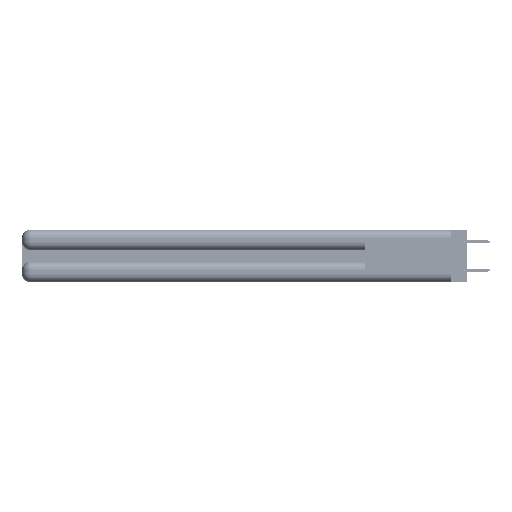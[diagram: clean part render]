
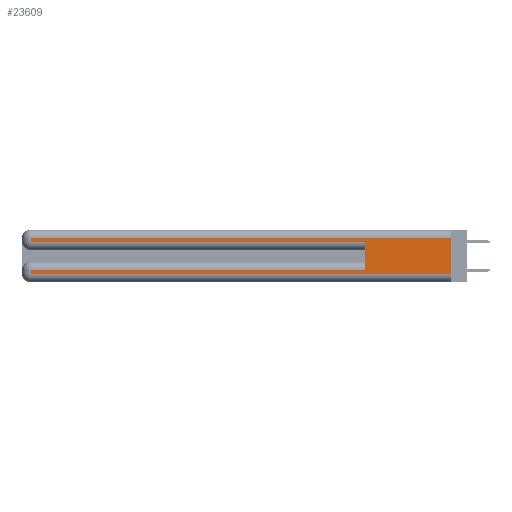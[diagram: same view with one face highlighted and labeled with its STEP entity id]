
A CAD part, left-side view. The second image highlights one B-rep face of the part: STEP entity #23609.
In plain terms, the highlighted planar face has unit normal (-1, 0, 0).
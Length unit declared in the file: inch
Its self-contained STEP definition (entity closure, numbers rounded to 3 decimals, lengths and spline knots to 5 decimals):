
#716 = DIRECTION ( 'NONE',  ( 0., 1., 0. ) ) ;
#971 = VECTOR ( 'NONE', #18711, 39.37008 ) ;
#2252 = LINE ( 'NONE', #43700, #971 ) ;
#2614 = CARTESIAN_POINT ( 'NONE',  ( 0., 0., 0.37 ) ) ;
#4484 = ORIENTED_EDGE ( 'NONE', *, *, #27002, .T. ) ;
#5103 = DIRECTION ( 'NONE',  ( 0., 0., -1. ) ) ;
#5315 = EDGE_CURVE ( 'NONE', #48750, #21793, #53080, .T. ) ;
#6388 = ORIENTED_EDGE ( 'NONE', *, *, #23982, .F. ) ;
#6727 = CARTESIAN_POINT ( 'NONE',  ( 0., 2.94, 0.285 ) ) ;
#11381 = DIRECTION ( 'NONE',  ( 0., 0., 1. ) ) ;
#13896 = LINE ( 'NONE', #39405, #26332 ) ;
#15158 = PLANE ( 'NONE',  #15555 ) ;
#15555 = AXIS2_PLACEMENT_3D ( 'NONE', #2614, #19742, #23743 ) ;
#15598 = EDGE_CURVE ( 'NONE', #36287, #19619, #33508, .T. ) ;
#16092 = LINE ( 'NONE', #33748, #53267 ) ;
#18470 = VECTOR ( 'NONE', #35921, 39.37008 ) ;
#18711 = DIRECTION ( 'NONE',  ( 0., 1., 0. ) ) ;
#18973 = EDGE_CURVE ( 'NONE', #51141, #25530, #16092, .T. ) ;
#19619 = VERTEX_POINT ( 'NONE', #25253 ) ;
#19698 = CARTESIAN_POINT ( 'NONE',  ( 0., 0., 0.06 ) ) ;
#19742 = DIRECTION ( 'NONE',  ( 1., 0., 0. ) ) ;
#20343 = ORIENTED_EDGE ( 'NONE', *, *, #15598, .T. ) ;
#21793 = VERTEX_POINT ( 'NONE', #26308 ) ;
#23037 = EDGE_CURVE ( 'NONE', #51141, #21793, #44058, .T. ) ;
#23609 = ADVANCED_FACE ( 'NONE', ( #45962 ), #15158, .F. ) ;
#23743 = DIRECTION ( 'NONE',  ( 0., 0., -1. ) ) ;
#23982 = EDGE_CURVE ( 'NONE', #47080, #19619, #13896, .T. ) ;
#25253 = CARTESIAN_POINT ( 'NONE',  ( 0., 0., 0.06 ) ) ;
#25530 = VERTEX_POINT ( 'NONE', #48719 ) ;
#26166 = CARTESIAN_POINT ( 'NONE',  ( 0., 0.6, 0.085 ) ) ;
#26308 = CARTESIAN_POINT ( 'NONE',  ( 0., 0.6, 0.285 ) ) ;
#26332 = VECTOR ( 'NONE', #51619, 39.37008 ) ;
#27002 = EDGE_CURVE ( 'NONE', #34077, #48750, #52098, .T. ) ;
#27604 = ORIENTED_EDGE ( 'NONE', *, *, #18973, .T. ) ;
#28381 = VECTOR ( 'NONE', #11381, 39.37008 ) ;
#28603 = VECTOR ( 'NONE', #49713, 39.37008 ) ;
#32104 = ORIENTED_EDGE ( 'NONE', *, *, #23037, .F. ) ;
#33508 = LINE ( 'NONE', #19698, #18470 ) ;
#33573 = ORIENTED_EDGE ( 'NONE', *, *, #38404, .T. ) ;
#33748 = CARTESIAN_POINT ( 'NONE',  ( 0., 0., 0.085 ) ) ;
#34077 = VERTEX_POINT ( 'NONE', #52692 ) ;
#35699 = VECTOR ( 'NONE', #5103, 39.37008 ) ;
#35862 = EDGE_LOOP ( 'NONE', ( #6388, #33573, #4484, #38631, #32104, #27604, #36655, #20343 ) ) ;
#35921 = DIRECTION ( 'NONE',  ( 0., -1., 0. ) ) ;
#36287 = VERTEX_POINT ( 'NONE', #50416 ) ;
#36388 = CARTESIAN_POINT ( 'NONE',  ( 0., 0.6, 0.145 ) ) ;
#36390 = CARTESIAN_POINT ( 'NONE',  ( 0., 0., 0.31 ) ) ;
#36655 = ORIENTED_EDGE ( 'NONE', *, *, #43906, .T. ) ;
#38404 = EDGE_CURVE ( 'NONE', #47080, #34077, #2252, .T. ) ;
#38631 = ORIENTED_EDGE ( 'NONE', *, *, #5315, .T. ) ;
#39405 = CARTESIAN_POINT ( 'NONE',  ( 0., 0., 0.37 ) ) ;
#41464 = DIRECTION ( 'NONE',  ( 0., -1., 0. ) ) ;
#42684 = VECTOR ( 'NONE', #41464, 39.37008 ) ;
#43700 = CARTESIAN_POINT ( 'NONE',  ( 0., 0., 0.31 ) ) ;
#43906 = EDGE_CURVE ( 'NONE', #25530, #36287, #52613, .T. ) ;
#44058 = LINE ( 'NONE', #36388, #28381 ) ;
#45962 = FACE_OUTER_BOUND ( 'NONE', #35862, .T. ) ;
#46347 = CARTESIAN_POINT ( 'NONE',  ( 0., 2.94, 0.37 ) ) ;
#47080 = VERTEX_POINT ( 'NONE', #36390 ) ;
#48719 = CARTESIAN_POINT ( 'NONE',  ( 0., 2.94, 0.085 ) ) ;
#48750 = VERTEX_POINT ( 'NONE', #6727 ) ;
#49525 = CARTESIAN_POINT ( 'NONE',  ( 0., 2.94, 0.37 ) ) ;
#49713 = DIRECTION ( 'NONE',  ( 0., 0., -1. ) ) ;
#50416 = CARTESIAN_POINT ( 'NONE',  ( 0., 2.94, 0.06 ) ) ;
#51141 = VERTEX_POINT ( 'NONE', #26166 ) ;
#51619 = DIRECTION ( 'NONE',  ( 0., 0., -1. ) ) ;
#52098 = LINE ( 'NONE', #49525, #28603 ) ;
#52613 = LINE ( 'NONE', #46347, #35699 ) ;
#52692 = CARTESIAN_POINT ( 'NONE',  ( 0., 2.94, 0.31 ) ) ;
#53080 = LINE ( 'NONE', #53622, #42684 ) ;
#53267 = VECTOR ( 'NONE', #716, 39.37008 ) ;
#53622 = CARTESIAN_POINT ( 'NONE',  ( 0., 0., 0.285 ) ) ;
